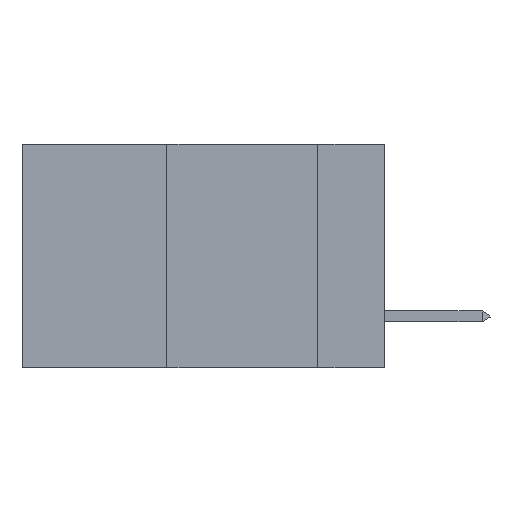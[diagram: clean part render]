
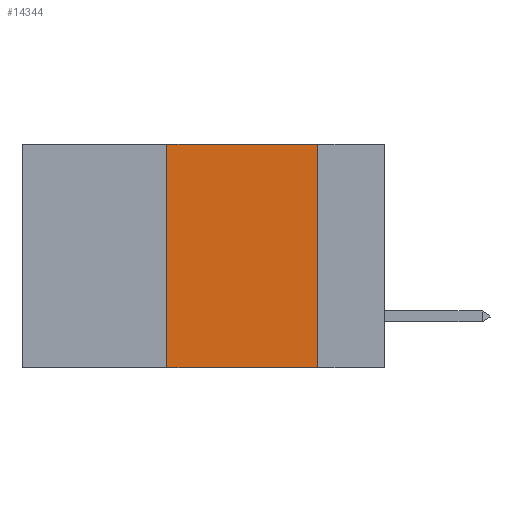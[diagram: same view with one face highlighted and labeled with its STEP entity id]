
A CAD part, left-side view. The second image highlights one B-rep face of the part: STEP entity #14344.
In plain terms, the highlighted planar face has unit normal (-1, 0, 0).
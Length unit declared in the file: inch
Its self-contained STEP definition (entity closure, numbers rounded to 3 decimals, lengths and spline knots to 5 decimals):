
#1785 = VERTEX_POINT ( 'NONE', #5578 ) ;
#1993 = VERTEX_POINT ( 'NONE', #24543 ) ;
#3248 = EDGE_CURVE ( 'NONE', #1785, #4341, #21761, .T. ) ;
#3469 = LINE ( 'NONE', #9731, #19541 ) ;
#4323 = CARTESIAN_POINT ( 'NONE',  ( 0., 0.6, 0. ) ) ;
#4341 = VERTEX_POINT ( 'NONE', #21342 ) ;
#5358 = AXIS2_PLACEMENT_3D ( 'NONE', #4323, #6487, #8314 ) ;
#5525 = DIRECTION ( 'NONE',  ( 0., 0., 1. ) ) ;
#5578 = CARTESIAN_POINT ( 'NONE',  ( 0., 0.11, 0. ) ) ;
#5974 = VECTOR ( 'NONE', #18646, 39.37008 ) ;
#6044 = CARTESIAN_POINT ( 'NONE',  ( 0., 0.36, 0. ) ) ;
#6487 = DIRECTION ( 'NONE',  ( 1., 0., 0. ) ) ;
#6745 = EDGE_CURVE ( 'NONE', #1993, #4341, #22297, .T. ) ;
#8314 = DIRECTION ( 'NONE',  ( 0., 0., -1. ) ) ;
#9200 = CARTESIAN_POINT ( 'NONE',  ( 0., 0.11, 0. ) ) ;
#9237 = EDGE_CURVE ( 'NONE', #11327, #1785, #15414, .T. ) ;
#9341 = CARTESIAN_POINT ( 'NONE',  ( 0., 0.6, -0.37 ) ) ;
#9482 = ORIENTED_EDGE ( 'NONE', *, *, #6745, .T. ) ;
#9731 = CARTESIAN_POINT ( 'NONE',  ( 0., 0.36, 0. ) ) ;
#11327 = VERTEX_POINT ( 'NONE', #6044 ) ;
#12145 = DIRECTION ( 'NONE',  ( 0., -1., 0. ) ) ;
#12182 = PLANE ( 'NONE',  #5358 ) ;
#12613 = VECTOR ( 'NONE', #12145, 39.37008 ) ;
#13088 = DIRECTION ( 'NONE',  ( 0., -1., 0. ) ) ;
#13420 = EDGE_CURVE ( 'NONE', #1993, #11327, #3469, .T. ) ;
#14344 = ADVANCED_FACE ( 'NONE', ( #18233 ), #12182, .F. ) ;
#14473 = EDGE_LOOP ( 'NONE', ( #16365, #18306, #16196, #9482 ) ) ;
#15414 = LINE ( 'NONE', #25053, #12613 ) ;
#16196 = ORIENTED_EDGE ( 'NONE', *, *, #13420, .F. ) ;
#16365 = ORIENTED_EDGE ( 'NONE', *, *, #3248, .F. ) ;
#17038 = VECTOR ( 'NONE', #13088, 39.37008 ) ;
#18233 = FACE_OUTER_BOUND ( 'NONE', #14473, .T. ) ;
#18306 = ORIENTED_EDGE ( 'NONE', *, *, #9237, .F. ) ;
#18646 = DIRECTION ( 'NONE',  ( 0., 0., -1. ) ) ;
#19541 = VECTOR ( 'NONE', #5525, 39.37008 ) ;
#21342 = CARTESIAN_POINT ( 'NONE',  ( 0., 0.11, -0.37 ) ) ;
#21761 = LINE ( 'NONE', #9200, #5974 ) ;
#22297 = LINE ( 'NONE', #9341, #17038 ) ;
#24543 = CARTESIAN_POINT ( 'NONE',  ( 0., 0.36, -0.37 ) ) ;
#25053 = CARTESIAN_POINT ( 'NONE',  ( 0., 0.6, 0. ) ) ;
